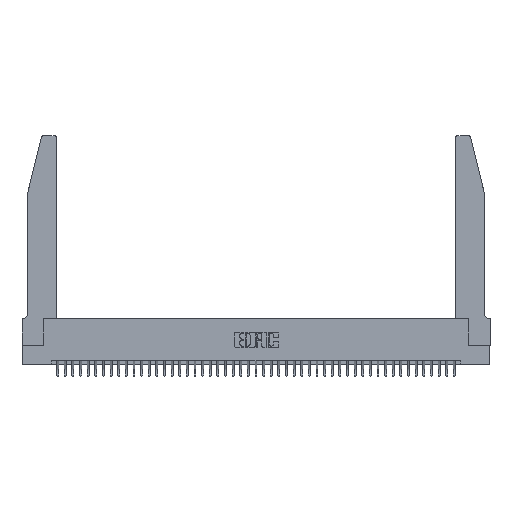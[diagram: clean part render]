
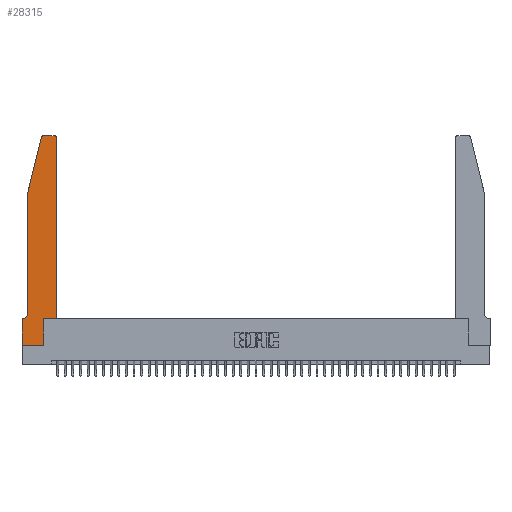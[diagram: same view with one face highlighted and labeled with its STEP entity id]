
A CAD part, top view. The second image highlights one B-rep face of the part: STEP entity #28315.
In plain terms, the highlighted planar face has unit normal (0, 0, 1).
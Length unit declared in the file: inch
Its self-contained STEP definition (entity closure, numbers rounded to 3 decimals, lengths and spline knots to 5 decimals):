
#879 = DIRECTION ( 'NONE',  ( 1., 0., 0. ) ) ;
#1554 = EDGE_CURVE ( 'NONE', #2955, #10228, #6824, .T. ) ;
#1617 = VECTOR ( 'NONE', #35564, 39.37008 ) ;
#1723 = CARTESIAN_POINT ( 'NONE',  ( 0., 0., 0.37 ) ) ;
#2955 = VERTEX_POINT ( 'NONE', #8041 ) ;
#2963 = VECTOR ( 'NONE', #3065, 39.37008 ) ;
#3065 = DIRECTION ( 'NONE',  ( 1., 0., 0. ) ) ;
#3125 = CARTESIAN_POINT ( 'NONE',  ( 0.0755, 2., 0.37 ) ) ;
#3233 = VECTOR ( 'NONE', #39963, 39.37008 ) ;
#4232 = CARTESIAN_POINT ( 'NONE',  ( 0., 0.35, 0.37 ) ) ;
#4513 = ORIENTED_EDGE ( 'NONE', *, *, #22986, .T. ) ;
#5251 = ORIENTED_EDGE ( 'NONE', *, *, #35093, .T. ) ;
#5477 = CARTESIAN_POINT ( 'NONE',  ( 0.4505, 0.35, 0.37 ) ) ;
#5551 = VERTEX_POINT ( 'NONE', #13064 ) ;
#6555 = CARTESIAN_POINT ( 'NONE',  ( 0.4205, 2.72, 0.37 ) ) ;
#6651 = DIRECTION ( 'NONE',  ( 0., -1., 0. ) ) ;
#6824 = LINE ( 'NONE', #20702, #32445 ) ;
#7381 = VERTEX_POINT ( 'NONE', #12680 ) ;
#7785 = VERTEX_POINT ( 'NONE', #44110 ) ;
#8041 = CARTESIAN_POINT ( 'NONE',  ( 0.0055, 0.35, 0.37 ) ) ;
#8269 = CARTESIAN_POINT ( 'NONE',  ( 0.2865, 0.35, 0.37 ) ) ;
#8772 = EDGE_CURVE ( 'NONE', #42426, #5551, #27870, .T. ) ;
#9109 = VERTEX_POINT ( 'NONE', #28014 ) ;
#10104 = ORIENTED_EDGE ( 'NONE', *, *, #19341, .T. ) ;
#10119 = DIRECTION ( 'NONE',  ( 1., 0., 0. ) ) ;
#10228 = VERTEX_POINT ( 'NONE', #29757 ) ;
#11409 = ORIENTED_EDGE ( 'NONE', *, *, #8772, .T. ) ;
#11428 = VECTOR ( 'NONE', #6651, 39.37008 ) ;
#11478 = VECTOR ( 'NONE', #26264, 39.37008 ) ;
#11838 = CARTESIAN_POINT ( 'NONE',  ( 0.0055, 0.42, 0.37 ) ) ;
#12114 = VERTEX_POINT ( 'NONE', #17864 ) ;
#12325 = EDGE_CURVE ( 'NONE', #40146, #30223, #31898, .T. ) ;
#12680 = CARTESIAN_POINT ( 'NONE',  ( 0., 0., 0.37 ) ) ;
#12818 = ORIENTED_EDGE ( 'NONE', *, *, #34226, .T. ) ;
#12982 = EDGE_CURVE ( 'NONE', #12114, #2955, #24890, .T. ) ;
#13064 = CARTESIAN_POINT ( 'NONE',  ( 0.4505, 2.72, 0.37 ) ) ;
#15322 = DIRECTION ( 'NONE',  ( -1., 0., 0. ) ) ;
#15340 = EDGE_LOOP ( 'NONE', ( #10104, #44039, #12818, #15497, #37222, #23601, #5251, #15958, #23297, #30688, #11409, #4513 ) ) ;
#15497 = ORIENTED_EDGE ( 'NONE', *, *, #34702, .T. ) ;
#15771 = CARTESIAN_POINT ( 'NONE',  ( 0.2605, 2.75, 0.37 ) ) ;
#15958 = ORIENTED_EDGE ( 'NONE', *, *, #19145, .T. ) ;
#16297 = AXIS2_PLACEMENT_3D ( 'NONE', #6555, #30925, #10119 ) ;
#17167 = CARTESIAN_POINT ( 'NONE',  ( 0.4505, 0.35, 0.37 ) ) ;
#17487 = LINE ( 'NONE', #1723, #26712 ) ;
#17864 = CARTESIAN_POINT ( 'NONE',  ( 0.0755, 0.42, 0.37 ) ) ;
#17993 = CARTESIAN_POINT ( 'NONE',  ( 0.2865, 0.35, 0.37 ) ) ;
#18916 = CARTESIAN_POINT ( 'NONE',  ( 0.284, 2.72, 0.37 ) ) ;
#18951 = LINE ( 'NONE', #32198, #1617 ) ;
#19145 = EDGE_CURVE ( 'NONE', #7381, #7785, #18951, .T. ) ;
#19341 = EDGE_CURVE ( 'NONE', #9109, #40146, #20774, .T. ) ;
#19571 = DIRECTION ( 'NONE',  ( 0., 1., 0. ) ) ;
#20025 = AXIS2_PLACEMENT_3D ( 'NONE', #11838, #36179, #15322 ) ;
#20500 = LINE ( 'NONE', #17167, #2963 ) ;
#20702 = CARTESIAN_POINT ( 'NONE',  ( 0.0755, 0.35, 0.37 ) ) ;
#20774 = LINE ( 'NONE', #15771, #11478 ) ;
#21493 = CARTESIAN_POINT ( 'NONE',  ( 0.0755, 2., 0.37 ) ) ;
#21497 = DIRECTION ( 'NONE',  ( 0., 1., 0. ) ) ;
#21834 = DIRECTION ( 'NONE',  ( 0., 0., 1. ) ) ;
#22409 = DIRECTION ( 'NONE',  ( 1., 0., 0. ) ) ;
#22975 = FACE_OUTER_BOUND ( 'NONE', #15340, .T. ) ;
#22986 = EDGE_CURVE ( 'NONE', #5551, #9109, #36718, .T. ) ;
#23297 = ORIENTED_EDGE ( 'NONE', *, *, #44666, .T. ) ;
#23601 = ORIENTED_EDGE ( 'NONE', *, *, #1554, .T. ) ;
#24055 = AXIS2_PLACEMENT_3D ( 'NONE', #18916, #43183, #22409 ) ;
#24295 = AXIS2_PLACEMENT_3D ( 'NONE', #4232, #21834, #879 ) ;
#24734 = CARTESIAN_POINT ( 'NONE',  ( 0.284, 2.75, 0.37 ) ) ;
#24890 = CIRCLE ( 'NONE', #20025, 0.07 ) ;
#26129 = DIRECTION ( 'NONE',  ( 0., -1., 0. ) ) ;
#26264 = DIRECTION ( 'NONE',  ( -1., 0., 0. ) ) ;
#26712 = VECTOR ( 'NONE', #26129, 39.37008 ) ;
#27870 = LINE ( 'NONE', #5477, #36048 ) ;
#28014 = CARTESIAN_POINT ( 'NONE',  ( 0.4205, 2.75, 0.37 ) ) ;
#28315 = ADVANCED_FACE ( 'NONE', ( #22975 ), #39148, .T. ) ;
#29115 = VERTEX_POINT ( 'NONE', #21493 ) ;
#29480 = CARTESIAN_POINT ( 'NONE',  ( 0.0755, 2., 0.37 ) ) ;
#29757 = CARTESIAN_POINT ( 'NONE',  ( 0., 0.35, 0.37 ) ) ;
#30223 = VERTEX_POINT ( 'NONE', #37654 ) ;
#30688 = ORIENTED_EDGE ( 'NONE', *, *, #41608, .T. ) ;
#30925 = DIRECTION ( 'NONE',  ( 0., 0., 1. ) ) ;
#30997 = LINE ( 'NONE', #3125, #11428 ) ;
#31898 = CIRCLE ( 'NONE', #24055, 0.03 ) ;
#32198 = CARTESIAN_POINT ( 'NONE',  ( 0., 0., 0.37 ) ) ;
#32445 = VECTOR ( 'NONE', #34648, 39.37008 ) ;
#32752 = VERTEX_POINT ( 'NONE', #8269 ) ;
#33636 = VECTOR ( 'NONE', #21497, 39.37008 ) ;
#34226 = EDGE_CURVE ( 'NONE', #30223, #29115, #40291, .T. ) ;
#34648 = DIRECTION ( 'NONE',  ( -1., 0., 0. ) ) ;
#34702 = EDGE_CURVE ( 'NONE', #29115, #12114, #30997, .T. ) ;
#34734 = LINE ( 'NONE', #17993, #33636 ) ;
#35093 = EDGE_CURVE ( 'NONE', #10228, #7381, #17487, .T. ) ;
#35466 = CARTESIAN_POINT ( 'NONE',  ( 0.4505, 0.35, 0.37 ) ) ;
#35564 = DIRECTION ( 'NONE',  ( 1., 0., 0. ) ) ;
#36048 = VECTOR ( 'NONE', #19571, 39.37008 ) ;
#36179 = DIRECTION ( 'NONE',  ( 0., 0., -1. ) ) ;
#36718 = CIRCLE ( 'NONE', #16297, 0.03 ) ;
#37222 = ORIENTED_EDGE ( 'NONE', *, *, #12982, .T. ) ;
#37654 = CARTESIAN_POINT ( 'NONE',  ( 0.25487, 2.72718, 0.37 ) ) ;
#39148 = PLANE ( 'NONE',  #24295 ) ;
#39963 = DIRECTION ( 'NONE',  ( -0.239, -0.971, 0. ) ) ;
#40146 = VERTEX_POINT ( 'NONE', #24734 ) ;
#40291 = LINE ( 'NONE', #29480, #3233 ) ;
#41608 = EDGE_CURVE ( 'NONE', #32752, #42426, #20500, .T. ) ;
#42426 = VERTEX_POINT ( 'NONE', #35466 ) ;
#43183 = DIRECTION ( 'NONE',  ( 0., 0., 1. ) ) ;
#44039 = ORIENTED_EDGE ( 'NONE', *, *, #12325, .T. ) ;
#44110 = CARTESIAN_POINT ( 'NONE',  ( 0.2865, 0., 0.37 ) ) ;
#44666 = EDGE_CURVE ( 'NONE', #7785, #32752, #34734, .T. ) ;
